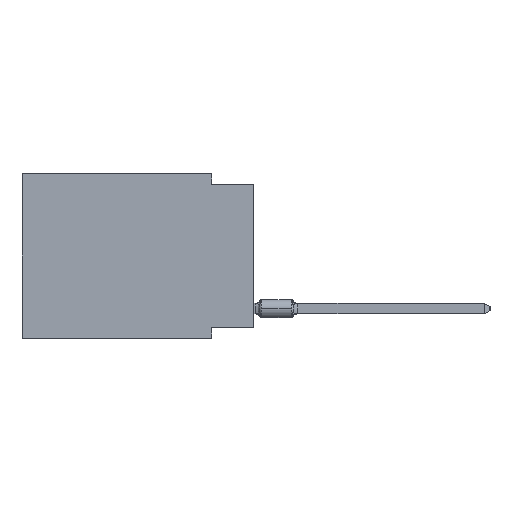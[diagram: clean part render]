
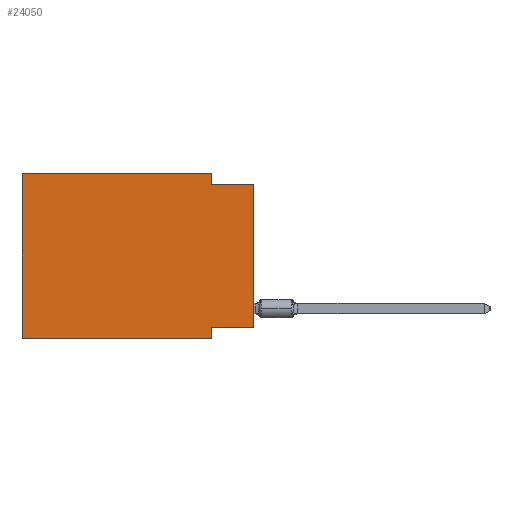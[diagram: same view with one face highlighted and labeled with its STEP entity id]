
A CAD part, left-side view. The second image highlights one B-rep face of the part: STEP entity #24050.
In plain terms, the highlighted planar face has unit normal (-1, 0, 0).
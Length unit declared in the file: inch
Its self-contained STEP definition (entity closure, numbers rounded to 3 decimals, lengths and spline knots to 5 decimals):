
#193 = CARTESIAN_POINT ( 'NONE',  ( 0., 0.1, -0.39 ) ) ;
#610 = ORIENTED_EDGE ( 'NONE', *, *, #1246, .F. ) ;
#699 = DIRECTION ( 'NONE',  ( 0., 1., 0. ) ) ;
#796 = ORIENTED_EDGE ( 'NONE', *, *, #15946, .F. ) ;
#912 = LINE ( 'NONE', #11897, #21787 ) ;
#1078 = ORIENTED_EDGE ( 'NONE', *, *, #25886, .T. ) ;
#1221 = DIRECTION ( 'NONE',  ( 0., 0., -1. ) ) ;
#1246 = EDGE_CURVE ( 'NONE', #21254, #9466, #2273, .T. ) ;
#1849 = LINE ( 'NONE', #23273, #11171 ) ;
#2273 = LINE ( 'NONE', #13396, #3393 ) ;
#2316 = VERTEX_POINT ( 'NONE', #3843 ) ;
#2961 = CARTESIAN_POINT ( 'NONE',  ( 0., 0.1, 0. ) ) ;
#3327 = DIRECTION ( 'NONE',  ( 1., 0., 0. ) ) ;
#3393 = VECTOR ( 'NONE', #19452, 39.37008 ) ;
#3799 = ORIENTED_EDGE ( 'NONE', *, *, #17483, .F. ) ;
#3843 = CARTESIAN_POINT ( 'NONE',  ( 0., 0.1, -0.365 ) ) ;
#4027 = LINE ( 'NONE', #23202, #6696 ) ;
#4469 = ORIENTED_EDGE ( 'NONE', *, *, #26318, .F. ) ;
#4833 = DIRECTION ( 'NONE',  ( 0., 0., 1. ) ) ;
#4893 = CARTESIAN_POINT ( 'NONE',  ( 0., 0.1, 0. ) ) ;
#4968 = LINE ( 'NONE', #17775, #24404 ) ;
#5487 = EDGE_CURVE ( 'NONE', #23065, #25092, #4027, .T. ) ;
#6305 = EDGE_CURVE ( 'NONE', #12569, #19777, #1849, .T. ) ;
#6696 = VECTOR ( 'NONE', #10642, 39.37008 ) ;
#7085 = CARTESIAN_POINT ( 'NONE',  ( 0., 0.55, 0. ) ) ;
#7181 = CARTESIAN_POINT ( 'NONE',  ( 0., 0.1, -0.39 ) ) ;
#7697 = CARTESIAN_POINT ( 'NONE',  ( 0., 0.55, 0. ) ) ;
#7967 = CARTESIAN_POINT ( 'NONE',  ( 0., 0., -0.025 ) ) ;
#8037 = EDGE_LOOP ( 'NONE', ( #1078, #610, #796, #21078, #3799, #16367, #17401, #4469 ) ) ;
#9466 = VERTEX_POINT ( 'NONE', #7967 ) ;
#9799 = VECTOR ( 'NONE', #13486, 39.37008 ) ;
#10367 = PLANE ( 'NONE',  #23871 ) ;
#10440 = CARTESIAN_POINT ( 'NONE',  ( 0., 0., -0.365 ) ) ;
#10642 = DIRECTION ( 'NONE',  ( 0., -1., 0. ) ) ;
#11171 = VECTOR ( 'NONE', #12828, 39.37008 ) ;
#11354 = VECTOR ( 'NONE', #699, 39.37008 ) ;
#11617 = DIRECTION ( 'NONE',  ( 0., 0., 1. ) ) ;
#11897 = CARTESIAN_POINT ( 'NONE',  ( 0., 0.55, 0. ) ) ;
#12569 = VERTEX_POINT ( 'NONE', #7085 ) ;
#12706 = VERTEX_POINT ( 'NONE', #10440 ) ;
#12828 = DIRECTION ( 'NONE',  ( 0., -1., 0. ) ) ;
#13396 = CARTESIAN_POINT ( 'NONE',  ( 0., 0., -0.025 ) ) ;
#13486 = DIRECTION ( 'NONE',  ( 0., 0., -1. ) ) ;
#15680 = CARTESIAN_POINT ( 'NONE',  ( 0., 0.55, -0.39 ) ) ;
#15946 = EDGE_CURVE ( 'NONE', #19777, #21254, #17838, .T. ) ;
#16367 = ORIENTED_EDGE ( 'NONE', *, *, #5487, .T. ) ;
#17401 = ORIENTED_EDGE ( 'NONE', *, *, #20919, .F. ) ;
#17483 = EDGE_CURVE ( 'NONE', #23065, #12569, #912, .T. ) ;
#17775 = CARTESIAN_POINT ( 'NONE',  ( 0., 0., 0. ) ) ;
#17838 = LINE ( 'NONE', #4893, #9799 ) ;
#19452 = DIRECTION ( 'NONE',  ( 0., -1., 0. ) ) ;
#19777 = VERTEX_POINT ( 'NONE', #2961 ) ;
#19994 = LINE ( 'NONE', #26347, #11354 ) ;
#20919 = EDGE_CURVE ( 'NONE', #2316, #25092, #21899, .T. ) ;
#21078 = ORIENTED_EDGE ( 'NONE', *, *, #6305, .F. ) ;
#21254 = VERTEX_POINT ( 'NONE', #25422 ) ;
#21787 = VECTOR ( 'NONE', #11617, 39.37008 ) ;
#21899 = LINE ( 'NONE', #193, #23662 ) ;
#22636 = FACE_OUTER_BOUND ( 'NONE', #8037, .T. ) ;
#23065 = VERTEX_POINT ( 'NONE', #15680 ) ;
#23202 = CARTESIAN_POINT ( 'NONE',  ( 0., 0.55, -0.39 ) ) ;
#23273 = CARTESIAN_POINT ( 'NONE',  ( 0., 0.55, 0. ) ) ;
#23662 = VECTOR ( 'NONE', #23868, 39.37008 ) ;
#23868 = DIRECTION ( 'NONE',  ( 0., 0., -1. ) ) ;
#23871 = AXIS2_PLACEMENT_3D ( 'NONE', #7697, #3327, #1221 ) ;
#24050 = ADVANCED_FACE ( 'NONE', ( #22636 ), #10367, .F. ) ;
#24404 = VECTOR ( 'NONE', #4833, 39.37008 ) ;
#25092 = VERTEX_POINT ( 'NONE', #7181 ) ;
#25422 = CARTESIAN_POINT ( 'NONE',  ( 0., 0.1, -0.025 ) ) ;
#25886 = EDGE_CURVE ( 'NONE', #12706, #9466, #4968, .T. ) ;
#26318 = EDGE_CURVE ( 'NONE', #12706, #2316, #19994, .T. ) ;
#26347 = CARTESIAN_POINT ( 'NONE',  ( 0., 0., -0.365 ) ) ;
